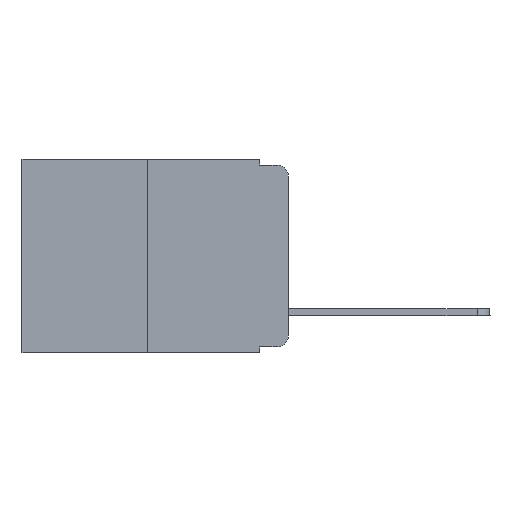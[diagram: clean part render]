
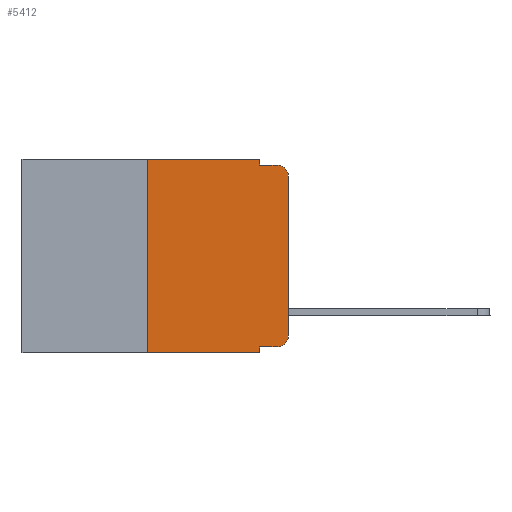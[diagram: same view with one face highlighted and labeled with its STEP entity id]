
A CAD part, left-side view. The second image highlights one B-rep face of the part: STEP entity #5412.
In plain terms, the highlighted planar face has unit normal (-1, 0, 0).
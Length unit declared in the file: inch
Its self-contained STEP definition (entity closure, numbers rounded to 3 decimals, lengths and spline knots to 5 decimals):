
#649 = VERTEX_POINT ( 'NONE', #12171 ) ;
#715 = EDGE_CURVE ( 'NONE', #3150, #7651, #5235, .T. ) ;
#738 = LINE ( 'NONE', #2632, #15230 ) ;
#1151 = CARTESIAN_POINT ( 'NONE',  ( 0., 0.25, 0. ) ) ;
#1193 = CARTESIAN_POINT ( 'NONE',  ( 0., 0.051, -0.333 ) ) ;
#1372 = CARTESIAN_POINT ( 'NONE',  ( 0., 0.02, -0.03 ) ) ;
#1380 = CARTESIAN_POINT ( 'NONE',  ( 0., 0.02, -0.313 ) ) ;
#1741 = CARTESIAN_POINT ( 'NONE',  ( 0., 0., -0.313 ) ) ;
#1869 = CIRCLE ( 'NONE', #4991, 0.02 ) ;
#2017 = ORIENTED_EDGE ( 'NONE', *, *, #19265, .T. ) ;
#2444 = VERTEX_POINT ( 'NONE', #1741 ) ;
#2632 = CARTESIAN_POINT ( 'NONE',  ( 0., 0.473, -0.343 ) ) ;
#2677 = LINE ( 'NONE', #9476, #6301 ) ;
#2714 = VECTOR ( 'NONE', #10848, 39.37008 ) ;
#2967 = DIRECTION ( 'NONE',  ( -1., 0., 0. ) ) ;
#3116 = VERTEX_POINT ( 'NONE', #16987 ) ;
#3150 = VERTEX_POINT ( 'NONE', #9010 ) ;
#3651 = ORIENTED_EDGE ( 'NONE', *, *, #13564, .T. ) ;
#4611 = AXIS2_PLACEMENT_3D ( 'NONE', #6048, #15451, #10716 ) ;
#4829 = CARTESIAN_POINT ( 'NONE',  ( 0., 0.473, 0. ) ) ;
#4938 = CARTESIAN_POINT ( 'NONE',  ( 0., 0.25, 0. ) ) ;
#4991 = AXIS2_PLACEMENT_3D ( 'NONE', #1380, #2967, #10565 ) ;
#5020 = CARTESIAN_POINT ( 'NONE',  ( 0., 0., -0.03 ) ) ;
#5235 = LINE ( 'NONE', #4938, #18889 ) ;
#5412 = ADVANCED_FACE ( 'NONE', ( #11480 ), #16931, .F. ) ;
#5512 = EDGE_CURVE ( 'NONE', #15360, #14648, #2677, .T. ) ;
#5661 = CARTESIAN_POINT ( 'NONE',  ( 0., 0.02, -0.01 ) ) ;
#6048 = CARTESIAN_POINT ( 'NONE',  ( 0., 0.473, 0. ) ) ;
#6301 = VECTOR ( 'NONE', #10783, 39.37008 ) ;
#6486 = EDGE_CURVE ( 'NONE', #649, #3116, #19247, .T. ) ;
#7074 = CARTESIAN_POINT ( 'NONE',  ( 0., 0., 0. ) ) ;
#7267 = VERTEX_POINT ( 'NONE', #8391 ) ;
#7651 = VERTEX_POINT ( 'NONE', #1151 ) ;
#7915 = ORIENTED_EDGE ( 'NONE', *, *, #17556, .F. ) ;
#8153 = ORIENTED_EDGE ( 'NONE', *, *, #5512, .F. ) ;
#8391 = CARTESIAN_POINT ( 'NONE',  ( 0., 0.051, 0. ) ) ;
#8753 = ORIENTED_EDGE ( 'NONE', *, *, #16780, .F. ) ;
#9010 = CARTESIAN_POINT ( 'NONE',  ( 0., 0.25, -0.343 ) ) ;
#9063 = ORIENTED_EDGE ( 'NONE', *, *, #715, .F. ) ;
#9476 = CARTESIAN_POINT ( 'NONE',  ( 0., 0.051, -0.01 ) ) ;
#9596 = ORIENTED_EDGE ( 'NONE', *, *, #19178, .F. ) ;
#10362 = DIRECTION ( 'NONE',  ( 0., 0., -1. ) ) ;
#10565 = DIRECTION ( 'NONE',  ( 0., 0., -1. ) ) ;
#10716 = DIRECTION ( 'NONE',  ( 0., 0., -1. ) ) ;
#10783 = DIRECTION ( 'NONE',  ( 0., -1., 0. ) ) ;
#10848 = DIRECTION ( 'NONE',  ( 0., 0., -1. ) ) ;
#10958 = VECTOR ( 'NONE', #12278, 39.37008 ) ;
#11480 = FACE_OUTER_BOUND ( 'NONE', #19177, .T. ) ;
#11506 = DIRECTION ( 'NONE',  ( 0., 0., 1. ) ) ;
#11809 = CARTESIAN_POINT ( 'NONE',  ( 0., 0.051, -0.343 ) ) ;
#11861 = DIRECTION ( 'NONE',  ( 0., -1., 0. ) ) ;
#12107 = ORIENTED_EDGE ( 'NONE', *, *, #6486, .T. ) ;
#12171 = CARTESIAN_POINT ( 'NONE',  ( 0., 0.051, -0.333 ) ) ;
#12278 = DIRECTION ( 'NONE',  ( 0., -1., 0. ) ) ;
#12311 = CIRCLE ( 'NONE', #17335, 0.02 ) ;
#12772 = DIRECTION ( 'NONE',  ( 0., 0., 1. ) ) ;
#12777 = ORIENTED_EDGE ( 'NONE', *, *, #16383, .T. ) ;
#12877 = VERTEX_POINT ( 'NONE', #5020 ) ;
#13035 = VECTOR ( 'NONE', #11506, 39.37008 ) ;
#13059 = LINE ( 'NONE', #15229, #18888 ) ;
#13315 = ORIENTED_EDGE ( 'NONE', *, *, #15686, .T. ) ;
#13564 = EDGE_CURVE ( 'NONE', #3116, #2444, #1869, .T. ) ;
#13705 = DIRECTION ( 'NONE',  ( 0., 0., -1. ) ) ;
#13994 = CARTESIAN_POINT ( 'NONE',  ( 0., 0.051, 0. ) ) ;
#14648 = VERTEX_POINT ( 'NONE', #5661 ) ;
#14752 = LINE ( 'NONE', #7074, #13035 ) ;
#15229 = CARTESIAN_POINT ( 'NONE',  ( 0., 0.051, 0. ) ) ;
#15230 = VECTOR ( 'NONE', #11861, 39.37008 ) ;
#15360 = VERTEX_POINT ( 'NONE', #16725 ) ;
#15451 = DIRECTION ( 'NONE',  ( 1., 0., 0. ) ) ;
#15686 = EDGE_CURVE ( 'NONE', #2444, #12877, #14752, .T. ) ;
#15749 = DIRECTION ( 'NONE',  ( 0., -1., 0. ) ) ;
#16383 = EDGE_CURVE ( 'NONE', #3150, #18463, #738, .T. ) ;
#16725 = CARTESIAN_POINT ( 'NONE',  ( 0., 0.051, -0.01 ) ) ;
#16780 = EDGE_CURVE ( 'NONE', #649, #18463, #17138, .T. ) ;
#16931 = PLANE ( 'NONE',  #4611 ) ;
#16987 = CARTESIAN_POINT ( 'NONE',  ( 0., 0.02, -0.333 ) ) ;
#17033 = DIRECTION ( 'NONE',  ( -1., 0., 0. ) ) ;
#17138 = LINE ( 'NONE', #13994, #2714 ) ;
#17335 = AXIS2_PLACEMENT_3D ( 'NONE', #1372, #17033, #13705 ) ;
#17556 = EDGE_CURVE ( 'NONE', #7651, #7267, #19472, .T. ) ;
#18002 = VECTOR ( 'NONE', #15749, 39.37008 ) ;
#18463 = VERTEX_POINT ( 'NONE', #11809 ) ;
#18888 = VECTOR ( 'NONE', #10362, 39.37008 ) ;
#18889 = VECTOR ( 'NONE', #12772, 39.37008 ) ;
#19177 = EDGE_LOOP ( 'NONE', ( #13315, #2017, #8153, #9596, #7915, #9063, #12777, #8753, #12107, #3651 ) ) ;
#19178 = EDGE_CURVE ( 'NONE', #7267, #15360, #13059, .T. ) ;
#19247 = LINE ( 'NONE', #1193, #10958 ) ;
#19265 = EDGE_CURVE ( 'NONE', #12877, #14648, #12311, .T. ) ;
#19472 = LINE ( 'NONE', #4829, #18002 ) ;
